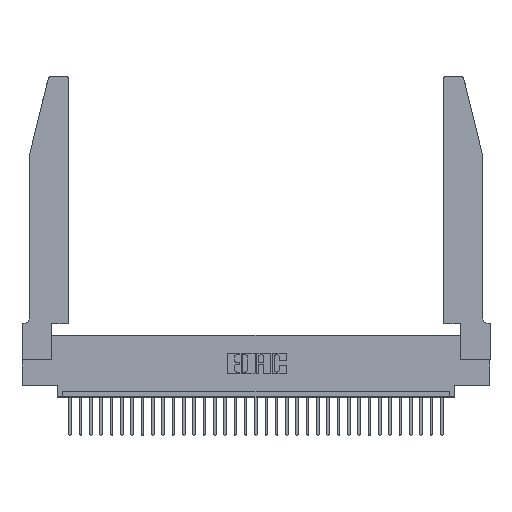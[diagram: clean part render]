
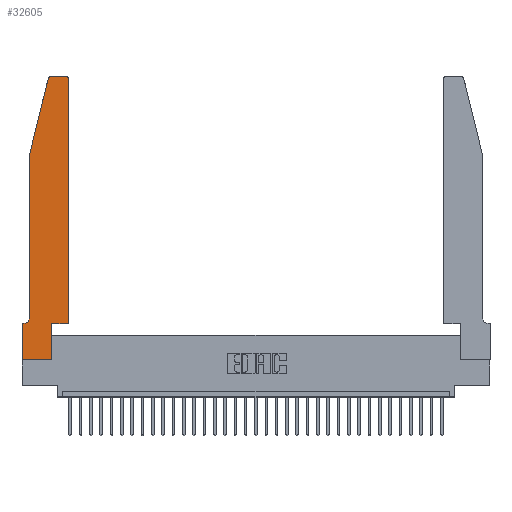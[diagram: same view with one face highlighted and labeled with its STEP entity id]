
A CAD part, top view. The second image highlights one B-rep face of the part: STEP entity #32605.
In plain terms, the highlighted planar face has unit normal (0, 0, 1).
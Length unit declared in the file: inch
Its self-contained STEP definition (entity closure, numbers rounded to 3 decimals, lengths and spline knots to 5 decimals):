
#589 = EDGE_LOOP ( 'NONE', ( #10246, #13371, #3102, #32870, #11254, #26936, #22954, #21175, #19259, #3824, #32186, #7402 ) ) ;
#601 = VERTEX_POINT ( 'NONE', #32591 ) ;
#828 = LINE ( 'NONE', #4813, #17384 ) ;
#894 = EDGE_CURVE ( 'NONE', #18856, #24506, #6351, .T. ) ;
#1601 = CIRCLE ( 'NONE', #5788, 0.07 ) ;
#1756 = FACE_OUTER_BOUND ( 'NONE', #589, .T. ) ;
#2846 = CARTESIAN_POINT ( 'NONE',  ( 0.0755, 2., 0.37 ) ) ;
#3014 = VERTEX_POINT ( 'NONE', #23161 ) ;
#3102 = ORIENTED_EDGE ( 'NONE', *, *, #6725, .T. ) ;
#3620 = LINE ( 'NONE', #31308, #14579 ) ;
#3824 = ORIENTED_EDGE ( 'NONE', *, *, #29164, .T. ) ;
#4813 = CARTESIAN_POINT ( 'NONE',  ( 0.4505, 0.35, 0.37 ) ) ;
#5093 = VERTEX_POINT ( 'NONE', #31470 ) ;
#5528 = VERTEX_POINT ( 'NONE', #28415 ) ;
#5606 = CARTESIAN_POINT ( 'NONE',  ( 0., 0., 0.37 ) ) ;
#5734 = DIRECTION ( 'NONE',  ( 0., -1., 0. ) ) ;
#5788 = AXIS2_PLACEMENT_3D ( 'NONE', #29544, #14140, #27177 ) ;
#6124 = EDGE_CURVE ( 'NONE', #18724, #601, #1601, .T. ) ;
#6250 = CARTESIAN_POINT ( 'NONE',  ( 0.4505, 0.35, 0.37 ) ) ;
#6351 = CIRCLE ( 'NONE', #29018, 0.03 ) ;
#6725 = EDGE_CURVE ( 'NONE', #24506, #9695, #11272, .T. ) ;
#7374 = DIRECTION ( 'NONE',  ( -1., 0., 0. ) ) ;
#7402 = ORIENTED_EDGE ( 'NONE', *, *, #30294, .T. ) ;
#9695 = VERTEX_POINT ( 'NONE', #27386 ) ;
#9962 = CARTESIAN_POINT ( 'NONE',  ( 0.284, 2.72, 0.37 ) ) ;
#10005 = PLANE ( 'NONE',  #12122 ) ;
#10246 = ORIENTED_EDGE ( 'NONE', *, *, #22148, .T. ) ;
#10363 = CARTESIAN_POINT ( 'NONE',  ( 0.4505, 0.35, 0.37 ) ) ;
#10882 = EDGE_CURVE ( 'NONE', #601, #22973, #11025, .T. ) ;
#11025 = LINE ( 'NONE', #15117, #15075 ) ;
#11205 = CARTESIAN_POINT ( 'NONE',  ( 0.2865, 0., 0.37 ) ) ;
#11254 = ORIENTED_EDGE ( 'NONE', *, *, #6124, .T. ) ;
#11272 = LINE ( 'NONE', #2846, #14513 ) ;
#12016 = VERTEX_POINT ( 'NONE', #6250 ) ;
#12122 = AXIS2_PLACEMENT_3D ( 'NONE', #25362, #22767, #15119 ) ;
#13371 = ORIENTED_EDGE ( 'NONE', *, *, #894, .T. ) ;
#13811 = VECTOR ( 'NONE', #31958, 39.37008 ) ;
#13916 = CARTESIAN_POINT ( 'NONE',  ( 0.0755, 2., 0.37 ) ) ;
#14140 = DIRECTION ( 'NONE',  ( 0., 0., -1. ) ) ;
#14454 = EDGE_CURVE ( 'NONE', #9695, #18724, #15005, .T. ) ;
#14513 = VECTOR ( 'NONE', #31068, 39.37008 ) ;
#14579 = VECTOR ( 'NONE', #23083, 39.37008 ) ;
#15005 = LINE ( 'NONE', #13916, #29137 ) ;
#15075 = VECTOR ( 'NONE', #33146, 39.37008 ) ;
#15117 = CARTESIAN_POINT ( 'NONE',  ( 0.0755, 0.35, 0.37 ) ) ;
#15119 = DIRECTION ( 'NONE',  ( 1., 0., 0. ) ) ;
#16085 = CARTESIAN_POINT ( 'NONE',  ( 0., 0.35, 0.37 ) ) ;
#17384 = VECTOR ( 'NONE', #20557, 39.37008 ) ;
#17785 = LINE ( 'NONE', #10363, #25426 ) ;
#17820 = CARTESIAN_POINT ( 'NONE',  ( 0.0755, 0.42, 0.37 ) ) ;
#17998 = VECTOR ( 'NONE', #31119, 39.37008 ) ;
#18192 = DIRECTION ( 'NONE',  ( 1., 0., 0. ) ) ;
#18236 = LINE ( 'NONE', #24733, #13811 ) ;
#18724 = VERTEX_POINT ( 'NONE', #17820 ) ;
#18856 = VERTEX_POINT ( 'NONE', #23657 ) ;
#19259 = ORIENTED_EDGE ( 'NONE', *, *, #22349, .T. ) ;
#20146 = EDGE_CURVE ( 'NONE', #22973, #20193, #23631, .T. ) ;
#20193 = VERTEX_POINT ( 'NONE', #5606 ) ;
#20557 = DIRECTION ( 'NONE',  ( 0., 1., 0. ) ) ;
#21175 = ORIENTED_EDGE ( 'NONE', *, *, #25924, .T. ) ;
#22148 = EDGE_CURVE ( 'NONE', #5528, #18856, #31530, .T. ) ;
#22349 = EDGE_CURVE ( 'NONE', #25764, #5093, #3620, .T. ) ;
#22767 = DIRECTION ( 'NONE',  ( 0., 0., 1. ) ) ;
#22954 = ORIENTED_EDGE ( 'NONE', *, *, #20146, .T. ) ;
#22973 = VERTEX_POINT ( 'NONE', #16085 ) ;
#23083 = DIRECTION ( 'NONE',  ( 0., 1., 0. ) ) ;
#23161 = CARTESIAN_POINT ( 'NONE',  ( 0.4505, 2.72, 0.37 ) ) ;
#23631 = LINE ( 'NONE', #28550, #17998 ) ;
#23657 = CARTESIAN_POINT ( 'NONE',  ( 0.284, 2.75, 0.37 ) ) ;
#23726 = CARTESIAN_POINT ( 'NONE',  ( 0.4205, 2.72, 0.37 ) ) ;
#24506 = VERTEX_POINT ( 'NONE', #32893 ) ;
#24733 = CARTESIAN_POINT ( 'NONE',  ( 0., 0., 0.37 ) ) ;
#25260 = AXIS2_PLACEMENT_3D ( 'NONE', #23726, #31512, #26228 ) ;
#25362 = CARTESIAN_POINT ( 'NONE',  ( 0., 0.35, 0.37 ) ) ;
#25426 = VECTOR ( 'NONE', #18192, 39.37008 ) ;
#25764 = VERTEX_POINT ( 'NONE', #11205 ) ;
#25924 = EDGE_CURVE ( 'NONE', #20193, #25764, #18236, .T. ) ;
#26228 = DIRECTION ( 'NONE',  ( 1., 0., 0. ) ) ;
#26936 = ORIENTED_EDGE ( 'NONE', *, *, #10882, .T. ) ;
#27177 = DIRECTION ( 'NONE',  ( -1., 0., 0. ) ) ;
#27386 = CARTESIAN_POINT ( 'NONE',  ( 0.0755, 2., 0.37 ) ) ;
#27581 = DIRECTION ( 'NONE',  ( 1., 0., 0. ) ) ;
#28415 = CARTESIAN_POINT ( 'NONE',  ( 0.4205, 2.75, 0.37 ) ) ;
#28550 = CARTESIAN_POINT ( 'NONE',  ( 0., 0., 0.37 ) ) ;
#28600 = DIRECTION ( 'NONE',  ( 0., 0., 1. ) ) ;
#28739 = EDGE_CURVE ( 'NONE', #12016, #3014, #828, .T. ) ;
#29018 = AXIS2_PLACEMENT_3D ( 'NONE', #9962, #28600, #27581 ) ;
#29137 = VECTOR ( 'NONE', #5734, 39.37008 ) ;
#29164 = EDGE_CURVE ( 'NONE', #5093, #12016, #17785, .T. ) ;
#29544 = CARTESIAN_POINT ( 'NONE',  ( 0.0055, 0.42, 0.37 ) ) ;
#30294 = EDGE_CURVE ( 'NONE', #3014, #5528, #30606, .T. ) ;
#30606 = CIRCLE ( 'NONE', #25260, 0.03 ) ;
#31068 = DIRECTION ( 'NONE',  ( -0.239, -0.971, 0. ) ) ;
#31101 = VECTOR ( 'NONE', #7374, 39.37008 ) ;
#31119 = DIRECTION ( 'NONE',  ( 0., -1., 0. ) ) ;
#31308 = CARTESIAN_POINT ( 'NONE',  ( 0.2865, 0.35, 0.37 ) ) ;
#31470 = CARTESIAN_POINT ( 'NONE',  ( 0.2865, 0.35, 0.37 ) ) ;
#31512 = DIRECTION ( 'NONE',  ( 0., 0., 1. ) ) ;
#31530 = LINE ( 'NONE', #33118, #31101 ) ;
#31958 = DIRECTION ( 'NONE',  ( 1., 0., 0. ) ) ;
#32186 = ORIENTED_EDGE ( 'NONE', *, *, #28739, .T. ) ;
#32591 = CARTESIAN_POINT ( 'NONE',  ( 0.0055, 0.35, 0.37 ) ) ;
#32605 = ADVANCED_FACE ( 'NONE', ( #1756 ), #10005, .T. ) ;
#32870 = ORIENTED_EDGE ( 'NONE', *, *, #14454, .T. ) ;
#32893 = CARTESIAN_POINT ( 'NONE',  ( 0.25487, 2.72718, 0.37 ) ) ;
#33118 = CARTESIAN_POINT ( 'NONE',  ( 0.2605, 2.75, 0.37 ) ) ;
#33146 = DIRECTION ( 'NONE',  ( -1., 0., 0. ) ) ;
